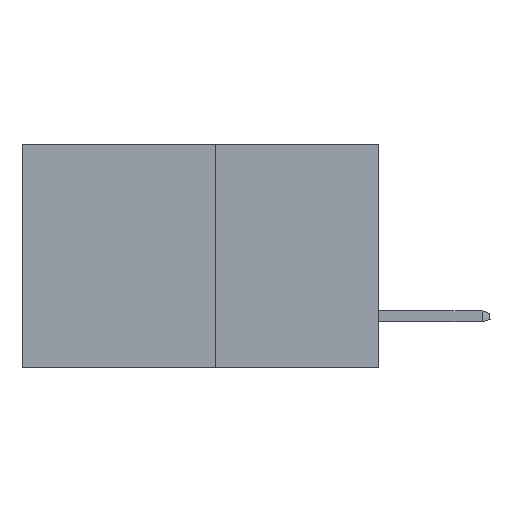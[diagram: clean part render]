
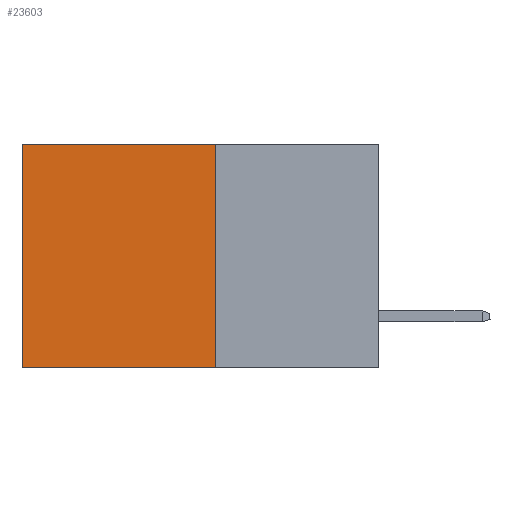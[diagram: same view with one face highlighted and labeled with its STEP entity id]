
A CAD part, left-side view. The second image highlights one B-rep face of the part: STEP entity #23603.
In plain terms, the highlighted planar face has unit normal (-1, 0, 0).
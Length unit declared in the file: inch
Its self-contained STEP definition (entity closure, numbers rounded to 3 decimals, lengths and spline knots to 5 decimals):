
#433 = CARTESIAN_POINT ( 'NONE',  ( 0.277, 0.27, -0.37 ) ) ;
#461 = EDGE_LOOP ( 'NONE', ( #10078, #18811, #15905, #1378 ) ) ;
#605 = CARTESIAN_POINT ( 'NONE',  ( 0.277, 0.27, -0.37 ) ) ;
#1378 = ORIENTED_EDGE ( 'NONE', *, *, #16185, .T. ) ;
#2004 = LINE ( 'NONE', #10769, #22149 ) ;
#2588 = DIRECTION ( 'NONE',  ( 1., 0., 0. ) ) ;
#2762 = CARTESIAN_POINT ( 'NONE',  ( 0.277, 0.59, -0.37 ) ) ;
#3460 = LINE ( 'NONE', #2762, #12705 ) ;
#4775 = DIRECTION ( 'NONE',  ( 0., 0., -1. ) ) ;
#4893 = CARTESIAN_POINT ( 'NONE',  ( 0.277, 0.59, -0.37 ) ) ;
#5708 = DIRECTION ( 'NONE',  ( 0., 1., 0. ) ) ;
#5939 = VERTEX_POINT ( 'NONE', #4893 ) ;
#6041 = EDGE_CURVE ( 'NONE', #22486, #5939, #2004, .T. ) ;
#6364 = CARTESIAN_POINT ( 'NONE',  ( 0.277, 0.27, 0. ) ) ;
#8097 = VERTEX_POINT ( 'NONE', #23687 ) ;
#9483 = DIRECTION ( 'NONE',  ( 0., 1., 0. ) ) ;
#10078 = ORIENTED_EDGE ( 'NONE', *, *, #22577, .T. ) ;
#10769 = CARTESIAN_POINT ( 'NONE',  ( 0.277, 0.27, -0.37 ) ) ;
#10960 = CARTESIAN_POINT ( 'NONE',  ( 0.277, 0.27, -0.37 ) ) ;
#11245 = VECTOR ( 'NONE', #22550, 39.37008 ) ;
#11872 = LINE ( 'NONE', #10960, #11245 ) ;
#12333 = FACE_OUTER_BOUND ( 'NONE', #461, .T. ) ;
#12705 = VECTOR ( 'NONE', #4775, 39.37008 ) ;
#13664 = AXIS2_PLACEMENT_3D ( 'NONE', #605, #2588, #16308 ) ;
#15390 = EDGE_CURVE ( 'NONE', #17739, #22486, #11872, .T. ) ;
#15905 = ORIENTED_EDGE ( 'NONE', *, *, #15390, .F. ) ;
#16185 = EDGE_CURVE ( 'NONE', #17739, #8097, #17571, .T. ) ;
#16308 = DIRECTION ( 'NONE',  ( 0., 0., -1. ) ) ;
#17376 = CARTESIAN_POINT ( 'NONE',  ( 0.277, 0.27, 0. ) ) ;
#17571 = LINE ( 'NONE', #17376, #23253 ) ;
#17739 = VERTEX_POINT ( 'NONE', #6364 ) ;
#18811 = ORIENTED_EDGE ( 'NONE', *, *, #6041, .F. ) ;
#22149 = VECTOR ( 'NONE', #9483, 39.37008 ) ;
#22486 = VERTEX_POINT ( 'NONE', #433 ) ;
#22550 = DIRECTION ( 'NONE',  ( 0., 0., -1. ) ) ;
#22577 = EDGE_CURVE ( 'NONE', #8097, #5939, #3460, .T. ) ;
#23253 = VECTOR ( 'NONE', #5708, 39.37008 ) ;
#23603 = ADVANCED_FACE ( 'NONE', ( #12333 ), #23923, .F. ) ;
#23687 = CARTESIAN_POINT ( 'NONE',  ( 0.277, 0.59, 0. ) ) ;
#23923 = PLANE ( 'NONE',  #13664 ) ;
